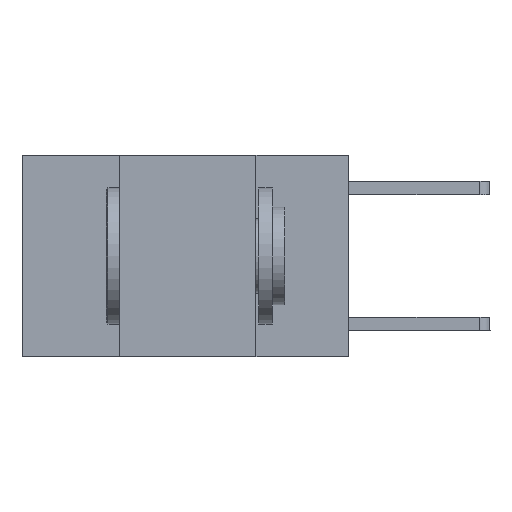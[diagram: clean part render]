
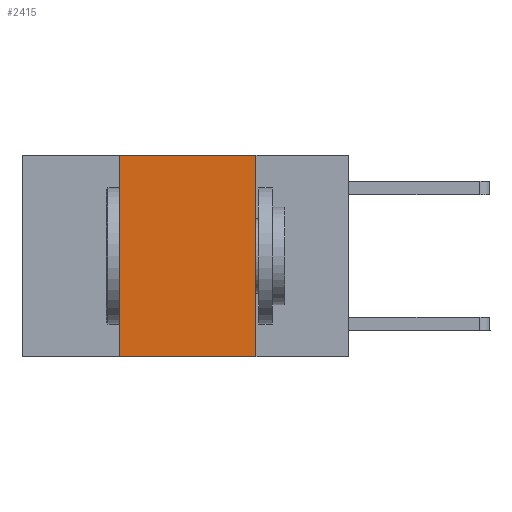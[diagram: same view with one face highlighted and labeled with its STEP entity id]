
A CAD part, left-side view. The second image highlights one B-rep face of the part: STEP entity #2415.
In plain terms, the highlighted planar face has unit normal (-1, 0, 0).
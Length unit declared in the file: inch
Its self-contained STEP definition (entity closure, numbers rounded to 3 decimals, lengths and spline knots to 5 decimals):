
#42 = CARTESIAN_POINT ( 'NONE',  ( 0., 0.6, 0. ) ) ;
#67 = DIRECTION ( 'NONE',  ( 1., 0., 0. ) ) ;
#72 = VECTOR ( 'NONE', #3502, 39.37008 ) ;
#1399 = CARTESIAN_POINT ( 'NONE',  ( 0., 0.17, -0.37 ) ) ;
#1571 = FACE_OUTER_BOUND ( 'NONE', #7241, .T. ) ;
#2415 = ADVANCED_FACE ( 'NONE', ( #1571 ), #8899, .F. ) ;
#2458 = CARTESIAN_POINT ( 'NONE',  ( 0., 0.6, 0. ) ) ;
#3502 = DIRECTION ( 'NONE',  ( 0., -1., 0. ) ) ;
#4387 = CARTESIAN_POINT ( 'NONE',  ( 0., 0.42, -0.37 ) ) ;
#4396 = AXIS2_PLACEMENT_3D ( 'NONE', #2458, #67, #8896 ) ;
#4813 = EDGE_CURVE ( 'NONE', #8930, #8531, #9097, .T. ) ;
#5020 = ORIENTED_EDGE ( 'NONE', *, *, #8240, .F. ) ;
#5145 = CARTESIAN_POINT ( 'NONE',  ( 0., 0.42, 0. ) ) ;
#5159 = DIRECTION ( 'NONE',  ( 0., -1., 0. ) ) ;
#5359 = ORIENTED_EDGE ( 'NONE', *, *, #8176, .F. ) ;
#5368 = EDGE_CURVE ( 'NONE', #8930, #8870, #10690, .T. ) ;
#5461 = VERTEX_POINT ( 'NONE', #9173 ) ;
#5668 = ORIENTED_EDGE ( 'NONE', *, *, #5368, .F. ) ;
#5675 = ORIENTED_EDGE ( 'NONE', *, *, #4813, .T. ) ;
#6100 = VECTOR ( 'NONE', #5159, 39.37008 ) ;
#6540 = CARTESIAN_POINT ( 'NONE',  ( 0., 0.42, 0. ) ) ;
#7241 = EDGE_LOOP ( 'NONE', ( #5020, #5359, #5668, #5675 ) ) ;
#7440 = DIRECTION ( 'NONE',  ( 0., 0., 1. ) ) ;
#7784 = CARTESIAN_POINT ( 'NONE',  ( 0., 0.17, 0. ) ) ;
#8176 = EDGE_CURVE ( 'NONE', #8870, #5461, #8393, .T. ) ;
#8240 = EDGE_CURVE ( 'NONE', #5461, #8531, #10511, .T. ) ;
#8393 = LINE ( 'NONE', #42, #6100 ) ;
#8531 = VERTEX_POINT ( 'NONE', #1399 ) ;
#8571 = VECTOR ( 'NONE', #7440, 39.37008 ) ;
#8589 = DIRECTION ( 'NONE',  ( 0., 0., -1. ) ) ;
#8870 = VERTEX_POINT ( 'NONE', #5145 ) ;
#8896 = DIRECTION ( 'NONE',  ( 0., 0., -1. ) ) ;
#8899 = PLANE ( 'NONE',  #4396 ) ;
#8930 = VERTEX_POINT ( 'NONE', #4387 ) ;
#9097 = LINE ( 'NONE', #9357, #72 ) ;
#9173 = CARTESIAN_POINT ( 'NONE',  ( 0., 0.17, 0. ) ) ;
#9357 = CARTESIAN_POINT ( 'NONE',  ( 0., 0.6, -0.37 ) ) ;
#10002 = VECTOR ( 'NONE', #8589, 39.37008 ) ;
#10511 = LINE ( 'NONE', #7784, #10002 ) ;
#10690 = LINE ( 'NONE', #6540, #8571 ) ;
